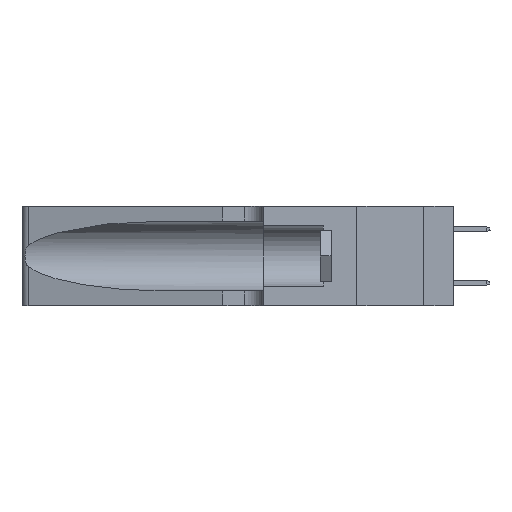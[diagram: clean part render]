
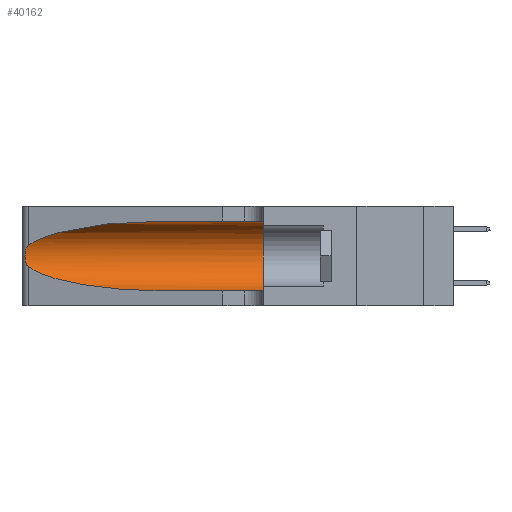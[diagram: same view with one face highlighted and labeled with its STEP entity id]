
A CAD part, left-side view. The second image highlights one B-rep face of the part: STEP entity #40162.
In plain terms, the highlighted cylindrical face has radius 3.308 mm (diameter 6.617 mm), a partial arc.
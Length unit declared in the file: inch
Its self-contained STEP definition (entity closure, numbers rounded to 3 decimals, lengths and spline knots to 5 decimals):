
#264 = EDGE_CURVE ( 'NONE', #32890, #30307, #34638, .T. ) ;
#513 = CARTESIAN_POINT ( 'NONE',  ( 0.25555, 1.22993, 0.14849 ) ) ;
#628 = AXIS2_PLACEMENT_3D ( 'NONE', #2714, #47741, #28425 ) ;
#1503 = CARTESIAN_POINT ( 'NONE',  ( 0.2373, 1.15595, 0.28018 ) ) ;
#2714 = CARTESIAN_POINT ( 'NONE',  ( 0.1305, 1.61858, 0.185 ) ) ;
#3944 = CARTESIAN_POINT ( 'NONE',  ( 0.1305, 0.35, 0.05475 ) ) ;
#4116 = CARTESIAN_POINT ( 'NONE',  ( 0.25487, 1.22718, 0.14631 ) ) ;
#4124 = EDGE_CURVE ( 'NONE', #32890, #18680, #32430, .T. ) ;
#5394 = CARTESIAN_POINT ( 'NONE',  ( 0.25487, 1.22718, 0.14631 ) ) ;
#5510 =( BOUNDED_CURVE ( )  B_SPLINE_CURVE ( 3, ( #5394, #20340, #20583, #35291 ),
 .UNSPECIFIED., .F., .T. ) 
 B_SPLINE_CURVE_WITH_KNOTS ( ( 4, 4 ),
 ( 3.44316, 4.71239 ),
 .UNSPECIFIED. ) 
 CURVE ( )  GEOMETRIC_REPRESENTATION_ITEM ( )  RATIONAL_B_SPLINE_CURVE ( ( 1., 0.87, 0.87, 1. ) ) 
 REPRESENTATION_ITEM ( '' )  );
#6660 = DIRECTION ( 'NONE',  ( 0., 1., 0. ) ) ;
#11277 = CARTESIAN_POINT ( 'NONE',  ( 0.25639, 1.23184, 0.21858 ) ) ;
#12384 = ORIENTED_EDGE ( 'NONE', *, *, #40018, .T. ) ;
#15431 = CARTESIAN_POINT ( 'NONE',  ( 0.25856, 1.23593, 0.16098 ) ) ;
#15687 = CARTESIAN_POINT ( 'NONE',  ( 0.1305, 0.72297, 0.31525 ) ) ;
#15777 = VECTOR ( 'NONE', #39482, 39.37008 ) ;
#16439 = CARTESIAN_POINT ( 'NONE',  ( 0.25487, 1.22718, 0.22369 ) ) ;
#16551 = AXIS2_PLACEMENT_3D ( 'NONE', #43885, #6660, #32872 ) ;
#17401 = CARTESIAN_POINT ( 'NONE',  ( 0.1305, 0.72297, 0.05475 ) ) ;
#18680 = VERTEX_POINT ( 'NONE', #38281 ) ;
#20340 = CARTESIAN_POINT ( 'NONE',  ( 0.2373, 1.15595, 0.08982 ) ) ;
#20414 = DIRECTION ( 'NONE',  ( 0., -1., 0. ) ) ;
#20583 = CARTESIAN_POINT ( 'NONE',  ( 0.18966, 0.96281, 0.05475 ) ) ;
#22775 = CARTESIAN_POINT ( 'NONE',  ( 0.25487, 1.22718, 0.14631 ) ) ;
#22789 = EDGE_CURVE ( 'NONE', #30307, #31659, #30623, .T. ) ;
#22811 = ORIENTED_EDGE ( 'NONE', *, *, #4124, .T. ) ;
#23032 = CARTESIAN_POINT ( 'NONE',  ( 0.25639, 1.23186, 0.15144 ) ) ;
#23858 = CARTESIAN_POINT ( 'NONE',  ( 0.1305, 1.61858, 0.31525 ) ) ;
#24940 = ORIENTED_EDGE ( 'NONE', *, *, #46693, .T. ) ;
#25264 = CARTESIAN_POINT ( 'NONE',  ( 0.25487, 1.22718, 0.22369 ) ) ;
#26228 = CARTESIAN_POINT ( 'NONE',  ( 0.26018, 1.23835, 0.19895 ) ) ;
#26961 = CARTESIAN_POINT ( 'NONE',  ( 0.18966, 0.96281, 0.31525 ) ) ;
#27823 = VERTEX_POINT ( 'NONE', #4116 ) ;
#28425 = DIRECTION ( 'NONE',  ( 0., 0., -1. ) ) ;
#29427 = CARTESIAN_POINT ( 'NONE',  ( 0.1305, 0.35, 0.31525 ) ) ;
#30307 = VERTEX_POINT ( 'NONE', #29427 ) ;
#30380 = EDGE_CURVE ( 'NONE', #18680, #27823, #35933, .T. ) ;
#30623 = CIRCLE ( 'NONE', #16551, 0.13025 ) ;
#31659 = VERTEX_POINT ( 'NONE', #3944 ) ;
#32430 =( BOUNDED_CURVE ( )  B_SPLINE_CURVE ( 3, ( #15687, #26961, #1503, #16439 ),
 .UNSPECIFIED., .F., .T. ) 
 B_SPLINE_CURVE_WITH_KNOTS ( ( 4, 4 ),
 ( 1.5708, 2.84003 ),
 .UNSPECIFIED. ) 
 CURVE ( )  GEOMETRIC_REPRESENTATION_ITEM ( )  RATIONAL_B_SPLINE_CURVE ( ( 1., 0.87, 0.87, 1. ) ) 
 REPRESENTATION_ITEM ( '' )  );
#32872 = DIRECTION ( 'NONE',  ( 0., 0., 1. ) ) ;
#32890 = VERTEX_POINT ( 'NONE', #44430 ) ;
#33563 = CARTESIAN_POINT ( 'NONE',  ( 0.25854, 1.2359, 0.20912 ) ) ;
#34638 = LINE ( 'NONE', #23858, #38627 ) ;
#35291 = CARTESIAN_POINT ( 'NONE',  ( 0.1305, 0.72297, 0.05475 ) ) ;
#35318 = VERTEX_POINT ( 'NONE', #17401 ) ;
#35786 = CYLINDRICAL_SURFACE ( 'NONE', #628, 0.13025 ) ;
#35933 = B_SPLINE_CURVE_WITH_KNOTS ( 'NONE', 3,
 ( #25264, #40902, #11277, #36533, #33563, #26228, #40187, #45300, #37719, #15431, #42355, #23032, #513, #22775 ),
 .UNSPECIFIED., .F., .F.,
 ( 4, 2, 2, 2, 2, 2, 4 ),
 ( 0., 0.00027, 0.00053, 0.00107, 0.0016, 0.00187, 0.00214 ),
 .UNSPECIFIED. ) ;
#36533 = CARTESIAN_POINT ( 'NONE',  ( 0.25787, 1.23484, 0.2124 ) ) ;
#37719 = CARTESIAN_POINT ( 'NONE',  ( 0.26017, 1.23833, 0.17102 ) ) ;
#38281 = CARTESIAN_POINT ( 'NONE',  ( 0.25487, 1.22718, 0.22369 ) ) ;
#38627 = VECTOR ( 'NONE', #20414, 39.37008 ) ;
#39482 = DIRECTION ( 'NONE',  ( 0., -1., 0. ) ) ;
#39725 = LINE ( 'NONE', #47557, #15777 ) ;
#40018 = EDGE_CURVE ( 'NONE', #27823, #35318, #5510, .T. ) ;
#40162 = ADVANCED_FACE ( 'NONE', ( #47012 ), #35786, .F. ) ;
#40187 = CARTESIAN_POINT ( 'NONE',  ( 0.26075, 1.23896, 0.19203 ) ) ;
#40902 = CARTESIAN_POINT ( 'NONE',  ( 0.25555, 1.22994, 0.2215 ) ) ;
#42355 = CARTESIAN_POINT ( 'NONE',  ( 0.25789, 1.23486, 0.15765 ) ) ;
#42409 = ORIENTED_EDGE ( 'NONE', *, *, #30380, .T. ) ;
#43885 = CARTESIAN_POINT ( 'NONE',  ( 0.1305, 0.35, 0.185 ) ) ;
#44212 = ORIENTED_EDGE ( 'NONE', *, *, #22789, .F. ) ;
#44430 = CARTESIAN_POINT ( 'NONE',  ( 0.1305, 0.72297, 0.31525 ) ) ;
#45300 = CARTESIAN_POINT ( 'NONE',  ( 0.26075, 1.23896, 0.178 ) ) ;
#46693 = EDGE_CURVE ( 'NONE', #35318, #31659, #39725, .T. ) ;
#47012 = FACE_OUTER_BOUND ( 'NONE', #47252, .T. ) ;
#47139 = ORIENTED_EDGE ( 'NONE', *, *, #264, .F. ) ;
#47252 = EDGE_LOOP ( 'NONE', ( #22811, #42409, #12384, #24940, #44212, #47139 ) ) ;
#47557 = CARTESIAN_POINT ( 'NONE',  ( 0.1305, 1.61858, 0.05475 ) ) ;
#47741 = DIRECTION ( 'NONE',  ( 0., -1., 0. ) ) ;
